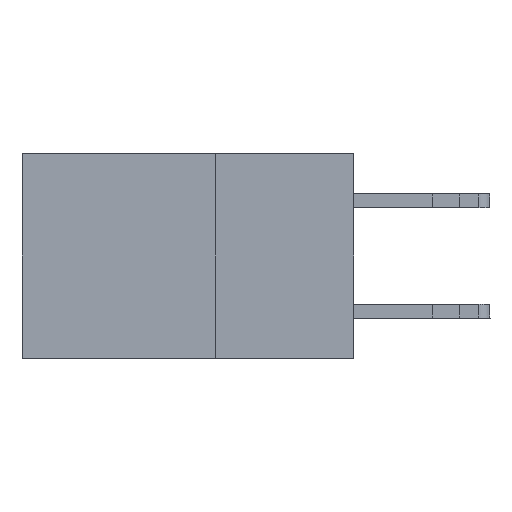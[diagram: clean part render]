
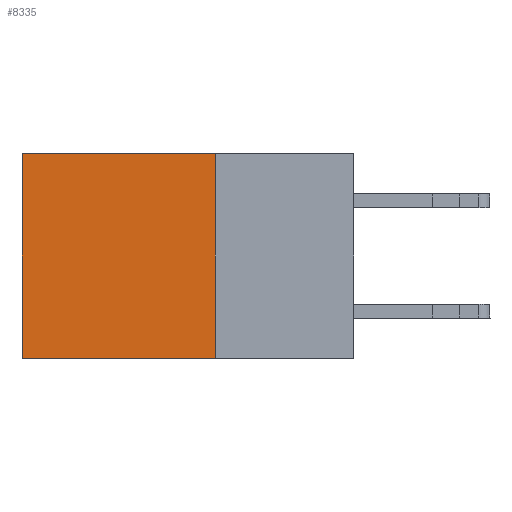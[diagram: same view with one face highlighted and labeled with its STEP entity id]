
A CAD part, left-side view. The second image highlights one B-rep face of the part: STEP entity #8335.
In plain terms, the highlighted planar face has unit normal (-1, 0, 0).
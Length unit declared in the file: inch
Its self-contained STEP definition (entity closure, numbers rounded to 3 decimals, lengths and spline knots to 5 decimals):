
#486 = VECTOR ( 'NONE', #8435, 39.37008 ) ;
#921 = CARTESIAN_POINT ( 'NONE',  ( 0.2875, 0.6, -0.37 ) ) ;
#2240 = VECTOR ( 'NONE', #17972, 39.37008 ) ;
#3147 = FACE_OUTER_BOUND ( 'NONE', #18096, .T. ) ;
#3335 = AXIS2_PLACEMENT_3D ( 'NONE', #5466, #17136, #7143 ) ;
#3775 = PLANE ( 'NONE',  #3335 ) ;
#3906 = CARTESIAN_POINT ( 'NONE',  ( 0.2875, 0.25, 0. ) ) ;
#4405 = LINE ( 'NONE', #10252, #21641 ) ;
#5466 = CARTESIAN_POINT ( 'NONE',  ( 0.2875, 0.25, 0. ) ) ;
#5993 = ORIENTED_EDGE ( 'NONE', *, *, #17411, .T. ) ;
#6098 = VERTEX_POINT ( 'NONE', #921 ) ;
#6690 = LINE ( 'NONE', #9666, #2240 ) ;
#6934 = DIRECTION ( 'NONE',  ( 0., 1., 0. ) ) ;
#7143 = DIRECTION ( 'NONE',  ( 0., 0., -1. ) ) ;
#8159 = EDGE_CURVE ( 'NONE', #12206, #16965, #20665, .T. ) ;
#8335 = ADVANCED_FACE ( 'NONE', ( #3147 ), #3775, .F. ) ;
#8435 = DIRECTION ( 'NONE',  ( 0., 1., 0. ) ) ;
#8452 = CARTESIAN_POINT ( 'NONE',  ( 0.2875, 0.25, -0.37 ) ) ;
#8735 = ORIENTED_EDGE ( 'NONE', *, *, #20093, .T. ) ;
#9666 = CARTESIAN_POINT ( 'NONE',  ( 0.2875, 0.6, 0. ) ) ;
#9995 = LINE ( 'NONE', #18413, #486 ) ;
#10252 = CARTESIAN_POINT ( 'NONE',  ( 0.2875, 0.25, -0.37 ) ) ;
#12206 = VERTEX_POINT ( 'NONE', #3906 ) ;
#12342 = ORIENTED_EDGE ( 'NONE', *, *, #20163, .F. ) ;
#13323 = DIRECTION ( 'NONE',  ( 0., 0., -1. ) ) ;
#13664 = ORIENTED_EDGE ( 'NONE', *, *, #8159, .F. ) ;
#16631 = CARTESIAN_POINT ( 'NONE',  ( 0.2875, 0.25, 0. ) ) ;
#16726 = VECTOR ( 'NONE', #13323, 39.37008 ) ;
#16965 = VERTEX_POINT ( 'NONE', #8452 ) ;
#17136 = DIRECTION ( 'NONE',  ( 1., 0., 0. ) ) ;
#17411 = EDGE_CURVE ( 'NONE', #19883, #6098, #6690, .T. ) ;
#17972 = DIRECTION ( 'NONE',  ( 0., 0., -1. ) ) ;
#18096 = EDGE_LOOP ( 'NONE', ( #5993, #12342, #13664, #8735 ) ) ;
#18413 = CARTESIAN_POINT ( 'NONE',  ( 0.2875, 0.25, 0. ) ) ;
#19294 = CARTESIAN_POINT ( 'NONE',  ( 0.2875, 0.6, 0. ) ) ;
#19883 = VERTEX_POINT ( 'NONE', #19294 ) ;
#20093 = EDGE_CURVE ( 'NONE', #12206, #19883, #9995, .T. ) ;
#20163 = EDGE_CURVE ( 'NONE', #16965, #6098, #4405, .T. ) ;
#20665 = LINE ( 'NONE', #16631, #16726 ) ;
#21641 = VECTOR ( 'NONE', #6934, 39.37008 ) ;
